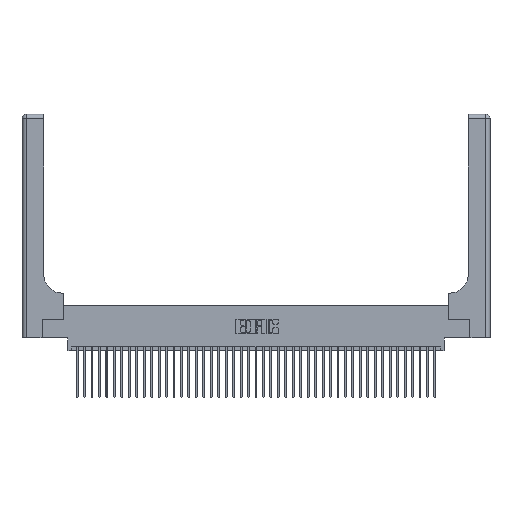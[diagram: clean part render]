
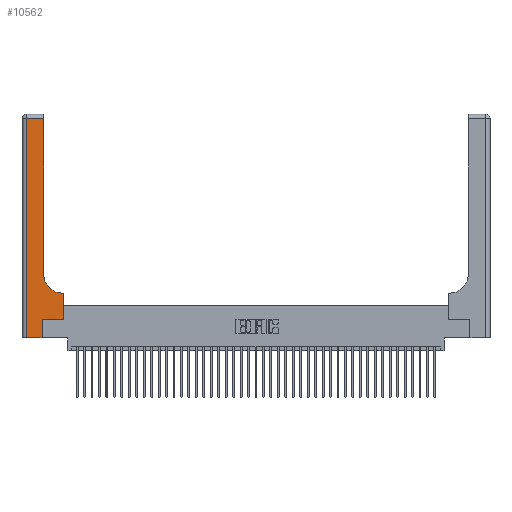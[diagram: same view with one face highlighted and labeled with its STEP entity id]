
A CAD part, top view. The second image highlights one B-rep face of the part: STEP entity #10562.
In plain terms, the highlighted planar face has unit normal (0, 0, 1).
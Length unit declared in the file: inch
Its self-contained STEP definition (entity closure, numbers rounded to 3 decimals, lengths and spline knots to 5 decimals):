
#207 = ORIENTED_EDGE ( 'NONE', *, *, #786, .T. ) ;
#664 = DIRECTION ( 'NONE',  ( 1., 0., 0. ) ) ;
#786 = EDGE_CURVE ( 'NONE', #17918, #35752, #25645, .T. ) ;
#1601 = DIRECTION ( 'NONE',  ( 1., 0., 0. ) ) ;
#2633 = ORIENTED_EDGE ( 'NONE', *, *, #9632, .T. ) ;
#4168 = LINE ( 'NONE', #4950, #42498 ) ;
#4182 = VECTOR ( 'NONE', #29392, 39.37008 ) ;
#4184 = CARTESIAN_POINT ( 'NONE',  ( 0.5585, 0.6, 0.37 ) ) ;
#4863 = EDGE_CURVE ( 'NONE', #35752, #4963, #26349, .T. ) ;
#4950 = CARTESIAN_POINT ( 'NONE',  ( 0.269, 0.25, 0.37 ) ) ;
#4963 = VERTEX_POINT ( 'NONE', #6276 ) ;
#5244 = LINE ( 'NONE', #14261, #21398 ) ;
#6124 = FACE_OUTER_BOUND ( 'NONE', #39818, .T. ) ;
#6263 = CARTESIAN_POINT ( 'NONE',  ( 0.2915, 3., 0.37 ) ) ;
#6276 = CARTESIAN_POINT ( 'NONE',  ( 0.06, 0., 0.37 ) ) ;
#6294 = LINE ( 'NONE', #35787, #4182 ) ;
#8357 = ORIENTED_EDGE ( 'NONE', *, *, #14133, .T. ) ;
#8432 = VERTEX_POINT ( 'NONE', #4184 ) ;
#9632 = EDGE_CURVE ( 'NONE', #34423, #24252, #9966, .T. ) ;
#9702 = CARTESIAN_POINT ( 'NONE',  ( 0.269, 0.25, 0.37 ) ) ;
#9966 = CIRCLE ( 'NONE', #36375, 0.25 ) ;
#10562 = ADVANCED_FACE ( 'NONE', ( #6124 ), #40275, .F. ) ;
#10671 = CARTESIAN_POINT ( 'NONE',  ( 0., 3., 0.37 ) ) ;
#10976 = EDGE_CURVE ( 'NONE', #4963, #16110, #18108, .T. ) ;
#12071 = CARTESIAN_POINT ( 'NONE',  ( 0.269, 0., 0.37 ) ) ;
#12856 = DIRECTION ( 'NONE',  ( 0., -1., 0. ) ) ;
#14002 = DIRECTION ( 'NONE',  ( 0., 0., -1. ) ) ;
#14133 = EDGE_CURVE ( 'NONE', #16110, #22137, #42715, .T. ) ;
#14261 = CARTESIAN_POINT ( 'NONE',  ( 0.2915, 0.6, 0.37 ) ) ;
#14348 = DIRECTION ( 'NONE',  ( 1., 0., 0. ) ) ;
#14774 = ORIENTED_EDGE ( 'NONE', *, *, #4863, .T. ) ;
#15232 = CARTESIAN_POINT ( 'NONE',  ( 0.269, 0., 0.37 ) ) ;
#15672 = DIRECTION ( 'NONE',  ( 0., 1., 0. ) ) ;
#16110 = VERTEX_POINT ( 'NONE', #15232 ) ;
#17918 = VERTEX_POINT ( 'NONE', #24189 ) ;
#18108 = LINE ( 'NONE', #34103, #33098 ) ;
#18342 = ORIENTED_EDGE ( 'NONE', *, *, #10976, .T. ) ;
#18840 = CARTESIAN_POINT ( 'NONE',  ( 0., 2.94, 0.37 ) ) ;
#19646 = VECTOR ( 'NONE', #26319, 39.37008 ) ;
#19899 = ORIENTED_EDGE ( 'NONE', *, *, #26346, .T. ) ;
#19901 = DIRECTION ( 'NONE',  ( 0., 0., -1. ) ) ;
#21338 = EDGE_CURVE ( 'NONE', #24252, #17918, #35105, .T. ) ;
#21398 = VECTOR ( 'NONE', #30611, 39.37008 ) ;
#22137 = VERTEX_POINT ( 'NONE', #9702 ) ;
#22380 = CARTESIAN_POINT ( 'NONE',  ( 0.5415, 0.85, 0.37 ) ) ;
#23305 = DIRECTION ( 'NONE',  ( -1., 0., 0. ) ) ;
#24189 = CARTESIAN_POINT ( 'NONE',  ( 0.2915, 2.94, 0.37 ) ) ;
#24252 = VERTEX_POINT ( 'NONE', #40609 ) ;
#25054 = CARTESIAN_POINT ( 'NONE',  ( 0.5415, 0.6, 0.37 ) ) ;
#25291 = VECTOR ( 'NONE', #12856, 39.37008 ) ;
#25313 = VERTEX_POINT ( 'NONE', #29690 ) ;
#25645 = LINE ( 'NONE', #18840, #41055 ) ;
#26265 = VECTOR ( 'NONE', #15672, 39.37008 ) ;
#26319 = DIRECTION ( 'NONE',  ( 0., 1., 0. ) ) ;
#26346 = EDGE_CURVE ( 'NONE', #22137, #25313, #4168, .T. ) ;
#26349 = LINE ( 'NONE', #28844, #25291 ) ;
#28844 = CARTESIAN_POINT ( 'NONE',  ( 0.06, 3., 0.37 ) ) ;
#29392 = DIRECTION ( 'NONE',  ( 0., 1., 0. ) ) ;
#29690 = CARTESIAN_POINT ( 'NONE',  ( 0.5585, 0.25, 0.37 ) ) ;
#30517 = ORIENTED_EDGE ( 'NONE', *, *, #35289, .T. ) ;
#30611 = DIRECTION ( 'NONE',  ( -1., 0., 0. ) ) ;
#32558 = AXIS2_PLACEMENT_3D ( 'NONE', #10671, #14002, #40417 ) ;
#33098 = VECTOR ( 'NONE', #14348, 39.37008 ) ;
#34103 = CARTESIAN_POINT ( 'NONE',  ( 0., 0., 0.37 ) ) ;
#34423 = VERTEX_POINT ( 'NONE', #25054 ) ;
#35105 = LINE ( 'NONE', #6263, #19646 ) ;
#35289 = EDGE_CURVE ( 'NONE', #8432, #34423, #5244, .T. ) ;
#35752 = VERTEX_POINT ( 'NONE', #39036 ) ;
#35787 = CARTESIAN_POINT ( 'NONE',  ( 0.5585, 0.25, 0.37 ) ) ;
#36375 = AXIS2_PLACEMENT_3D ( 'NONE', #22380, #19901, #664 ) ;
#38792 = ORIENTED_EDGE ( 'NONE', *, *, #21338, .T. ) ;
#39036 = CARTESIAN_POINT ( 'NONE',  ( 0.06, 2.94, 0.37 ) ) ;
#39818 = EDGE_LOOP ( 'NONE', ( #38792, #207, #14774, #18342, #8357, #19899, #41080, #30517, #2633 ) ) ;
#40275 = PLANE ( 'NONE',  #32558 ) ;
#40417 = DIRECTION ( 'NONE',  ( -1., 0., 0. ) ) ;
#40609 = CARTESIAN_POINT ( 'NONE',  ( 0.2915, 0.85, 0.37 ) ) ;
#41055 = VECTOR ( 'NONE', #23305, 39.37008 ) ;
#41080 = ORIENTED_EDGE ( 'NONE', *, *, #42264, .T. ) ;
#42264 = EDGE_CURVE ( 'NONE', #25313, #8432, #6294, .T. ) ;
#42498 = VECTOR ( 'NONE', #1601, 39.37008 ) ;
#42715 = LINE ( 'NONE', #12071, #26265 ) ;
